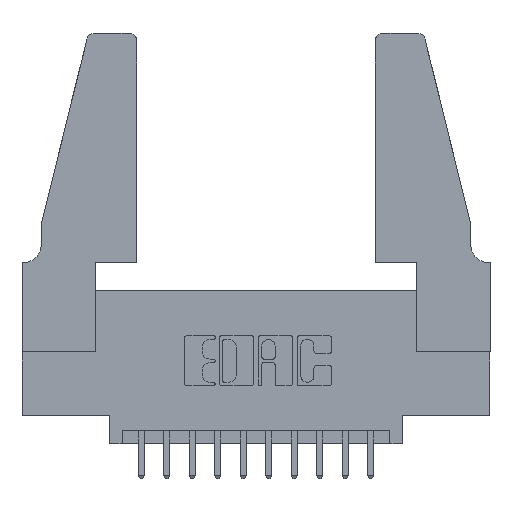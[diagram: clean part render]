
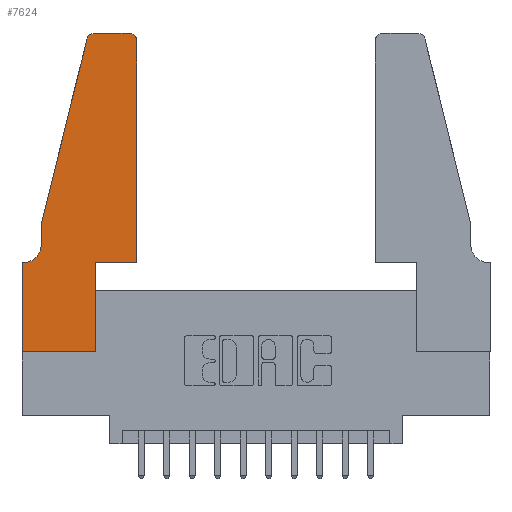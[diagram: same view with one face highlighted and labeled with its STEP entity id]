
A CAD part, top view. The second image highlights one B-rep face of the part: STEP entity #7624.
In plain terms, the highlighted planar face has unit normal (0, 0, 1).
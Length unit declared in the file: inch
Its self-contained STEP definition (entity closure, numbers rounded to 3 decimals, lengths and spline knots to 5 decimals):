
#226 = CARTESIAN_POINT ( 'NONE',  ( 0.4505, 1.22, 0.37 ) ) ;
#696 = DIRECTION ( 'NONE',  ( -1., 0., 0. ) ) ;
#720 = VERTEX_POINT ( 'NONE', #226 ) ;
#993 = LINE ( 'NONE', #3710, #4037 ) ;
#1036 = ORIENTED_EDGE ( 'NONE', *, *, #13344, .T. ) ;
#1322 = AXIS2_PLACEMENT_3D ( 'NONE', #1914, #9742, #3034 ) ;
#1352 = CARTESIAN_POINT ( 'NONE',  ( 0., 0., 0.37 ) ) ;
#1390 = ORIENTED_EDGE ( 'NONE', *, *, #13275, .T. ) ;
#1434 = PLANE ( 'NONE',  #5107 ) ;
#1488 = DIRECTION ( 'NONE',  ( 1., 0., 0. ) ) ;
#1508 = EDGE_CURVE ( 'NONE', #12283, #6649, #6121, .T. ) ;
#1560 = AXIS2_PLACEMENT_3D ( 'NONE', #8507, #1795, #9632 ) ;
#1659 = DIRECTION ( 'NONE',  ( 0., -1., 0. ) ) ;
#1795 = DIRECTION ( 'NONE',  ( 0., 0., 1. ) ) ;
#1893 = CARTESIAN_POINT ( 'NONE',  ( 0.284, 1.25, 0.37 ) ) ;
#1914 = CARTESIAN_POINT ( 'NONE',  ( 0.284, 1.22, 0.37 ) ) ;
#1966 = VERTEX_POINT ( 'NONE', #9335 ) ;
#2027 = AXIS2_PLACEMENT_3D ( 'NONE', #3265, #11071, #4432 ) ;
#2091 = EDGE_CURVE ( 'NONE', #5961, #3559, #11285, .T. ) ;
#2486 = CARTESIAN_POINT ( 'NONE',  ( 0.2865, 0.35, 0.37 ) ) ;
#2579 = CARTESIAN_POINT ( 'NONE',  ( 0., 0.35, 0.37 ) ) ;
#2581 = VECTOR ( 'NONE', #13269, 39.37008 ) ;
#2893 = LINE ( 'NONE', #13477, #14011 ) ;
#2992 = ORIENTED_EDGE ( 'NONE', *, *, #4532, .T. ) ;
#3034 = DIRECTION ( 'NONE',  ( 1., 0., 0. ) ) ;
#3116 = DIRECTION ( 'NONE',  ( -1., 0., 0. ) ) ;
#3265 = CARTESIAN_POINT ( 'NONE',  ( 0.0055, 0.42, 0.37 ) ) ;
#3494 = DIRECTION ( 'NONE',  ( 1., 0., 0. ) ) ;
#3559 = VERTEX_POINT ( 'NONE', #5637 ) ;
#3710 = CARTESIAN_POINT ( 'NONE',  ( 0.2865, 0.35, 0.37 ) ) ;
#3738 = DIRECTION ( 'NONE',  ( 1., 0., 0. ) ) ;
#4001 = CARTESIAN_POINT ( 'NONE',  ( 0.0755, 0.42, 0.37 ) ) ;
#4037 = VECTOR ( 'NONE', #10373, 39.37008 ) ;
#4413 = CIRCLE ( 'NONE', #1560, 0.03 ) ;
#4432 = DIRECTION ( 'NONE',  ( -1., 0., 0. ) ) ;
#4456 = ORIENTED_EDGE ( 'NONE', *, *, #5131, .T. ) ;
#4532 = EDGE_CURVE ( 'NONE', #720, #12727, #4413, .T. ) ;
#4806 = VECTOR ( 'NONE', #3116, 39.37008 ) ;
#4965 = EDGE_CURVE ( 'NONE', #6649, #14265, #993, .T. ) ;
#5107 = AXIS2_PLACEMENT_3D ( 'NONE', #2579, #10409, #3738 ) ;
#5131 = EDGE_CURVE ( 'NONE', #12173, #12283, #13381, .T. ) ;
#5190 = VERTEX_POINT ( 'NONE', #4001 ) ;
#5601 = CARTESIAN_POINT ( 'NONE',  ( 0.4505, 0.35, 0.37 ) ) ;
#5637 = CARTESIAN_POINT ( 'NONE',  ( 0.25487, 1.22718, 0.37 ) ) ;
#5961 = VERTEX_POINT ( 'NONE', #1893 ) ;
#6121 = LINE ( 'NONE', #10846, #11981 ) ;
#6144 = EDGE_CURVE ( 'NONE', #1966, #720, #11475, .T. ) ;
#6165 = CARTESIAN_POINT ( 'NONE',  ( 0., 0., 0.37 ) ) ;
#6247 = CARTESIAN_POINT ( 'NONE',  ( 0.0755, 0.5, 0.37 ) ) ;
#6480 = CARTESIAN_POINT ( 'NONE',  ( 0.0755, 0.5, 0.37 ) ) ;
#6595 = CARTESIAN_POINT ( 'NONE',  ( 0.0055, 0.35, 0.37 ) ) ;
#6649 = VERTEX_POINT ( 'NONE', #10801 ) ;
#6696 = CARTESIAN_POINT ( 'NONE',  ( 0.4205, 1.25, 0.37 ) ) ;
#6809 = CARTESIAN_POINT ( 'NONE',  ( 0., 0.35, 0.37 ) ) ;
#6919 = LINE ( 'NONE', #6247, #7251 ) ;
#6968 = ORIENTED_EDGE ( 'NONE', *, *, #2091, .T. ) ;
#7074 = CIRCLE ( 'NONE', #2027, 0.07 ) ;
#7251 = VECTOR ( 'NONE', #13936, 39.37008 ) ;
#7286 = VERTEX_POINT ( 'NONE', #6595 ) ;
#7459 = CARTESIAN_POINT ( 'NONE',  ( 0.0755, 0.35, 0.37 ) ) ;
#7503 = EDGE_CURVE ( 'NONE', #14265, #1966, #2893, .T. ) ;
#7512 = VECTOR ( 'NONE', #1659, 39.37008 ) ;
#7624 = ADVANCED_FACE ( 'NONE', ( #9367 ), #1434, .T. ) ;
#7904 = EDGE_CURVE ( 'NONE', #14159, #5190, #8833, .T. ) ;
#8390 = ORIENTED_EDGE ( 'NONE', *, *, #7904, .T. ) ;
#8489 = VECTOR ( 'NONE', #13032, 39.37008 ) ;
#8507 = CARTESIAN_POINT ( 'NONE',  ( 0.4205, 1.22, 0.37 ) ) ;
#8643 = LINE ( 'NONE', #7459, #14155 ) ;
#8833 = LINE ( 'NONE', #6480, #8489 ) ;
#9153 = ORIENTED_EDGE ( 'NONE', *, *, #13128, .T. ) ;
#9335 = CARTESIAN_POINT ( 'NONE',  ( 0.4505, 0.35, 0.37 ) ) ;
#9367 = FACE_OUTER_BOUND ( 'NONE', #13641, .T. ) ;
#9632 = DIRECTION ( 'NONE',  ( 1., 0., 0. ) ) ;
#9742 = DIRECTION ( 'NONE',  ( 0., 0., 1. ) ) ;
#10373 = DIRECTION ( 'NONE',  ( 0., 1., 0. ) ) ;
#10409 = DIRECTION ( 'NONE',  ( 0., 0., 1. ) ) ;
#10541 = ORIENTED_EDGE ( 'NONE', *, *, #6144, .T. ) ;
#10700 = LINE ( 'NONE', #12019, #4806 ) ;
#10801 = CARTESIAN_POINT ( 'NONE',  ( 0.2865, 0., 0.37 ) ) ;
#10846 = CARTESIAN_POINT ( 'NONE',  ( 0., 0., 0.37 ) ) ;
#10988 = CARTESIAN_POINT ( 'NONE',  ( 0.0755, 0.5, 0.37 ) ) ;
#11071 = DIRECTION ( 'NONE',  ( 0., 0., -1. ) ) ;
#11196 = ORIENTED_EDGE ( 'NONE', *, *, #12509, .T. ) ;
#11271 = ORIENTED_EDGE ( 'NONE', *, *, #7503, .T. ) ;
#11285 = CIRCLE ( 'NONE', #1322, 0.03 ) ;
#11475 = LINE ( 'NONE', #5601, #2581 ) ;
#11607 = ORIENTED_EDGE ( 'NONE', *, *, #1508, .T. ) ;
#11981 = VECTOR ( 'NONE', #1488, 39.37008 ) ;
#12019 = CARTESIAN_POINT ( 'NONE',  ( 0.2605, 1.25, 0.37 ) ) ;
#12173 = VERTEX_POINT ( 'NONE', #6809 ) ;
#12283 = VERTEX_POINT ( 'NONE', #1352 ) ;
#12509 = EDGE_CURVE ( 'NONE', #7286, #12173, #8643, .T. ) ;
#12727 = VERTEX_POINT ( 'NONE', #6696 ) ;
#13032 = DIRECTION ( 'NONE',  ( 0., -1., 0. ) ) ;
#13128 = EDGE_CURVE ( 'NONE', #3559, #14159, #6919, .T. ) ;
#13175 = ORIENTED_EDGE ( 'NONE', *, *, #4965, .T. ) ;
#13269 = DIRECTION ( 'NONE',  ( 0., 1., 0. ) ) ;
#13275 = EDGE_CURVE ( 'NONE', #12727, #5961, #10700, .T. ) ;
#13344 = EDGE_CURVE ( 'NONE', #5190, #7286, #7074, .T. ) ;
#13381 = LINE ( 'NONE', #6165, #7512 ) ;
#13477 = CARTESIAN_POINT ( 'NONE',  ( 0.4505, 0.35, 0.37 ) ) ;
#13641 = EDGE_LOOP ( 'NONE', ( #1390, #6968, #9153, #8390, #1036, #11196, #4456, #11607, #13175, #11271, #10541, #2992 ) ) ;
#13936 = DIRECTION ( 'NONE',  ( -0.239, -0.971, 0. ) ) ;
#14011 = VECTOR ( 'NONE', #3494, 39.37008 ) ;
#14155 = VECTOR ( 'NONE', #696, 39.37008 ) ;
#14159 = VERTEX_POINT ( 'NONE', #10988 ) ;
#14265 = VERTEX_POINT ( 'NONE', #2486 ) ;
